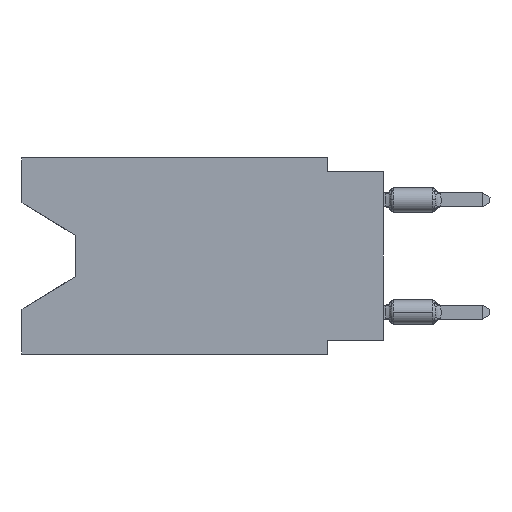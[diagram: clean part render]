
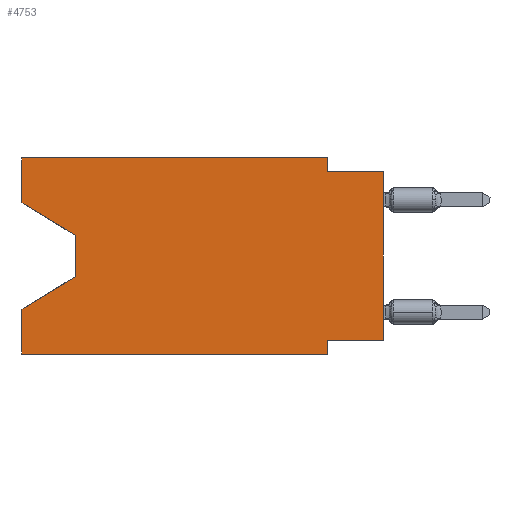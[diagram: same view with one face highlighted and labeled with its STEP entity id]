
A CAD part, left-side view. The second image highlights one B-rep face of the part: STEP entity #4753.
In plain terms, the highlighted planar face has unit normal (-1, 0, 0).
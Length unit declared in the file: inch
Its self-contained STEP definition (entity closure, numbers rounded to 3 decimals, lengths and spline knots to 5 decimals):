
#334 = ORIENTED_EDGE ( 'NONE', *, *, #19707, .F. ) ;
#406 = LINE ( 'NONE', #18886, #5684 ) ;
#440 = ORIENTED_EDGE ( 'NONE', *, *, #2160, .T. ) ;
#480 = VECTOR ( 'NONE', #18942, 39.37008 ) ;
#954 = VERTEX_POINT ( 'NONE', #6726 ) ;
#1253 = ORIENTED_EDGE ( 'NONE', *, *, #10265, .T. ) ;
#1582 = VERTEX_POINT ( 'NONE', #18762 ) ;
#1599 = DIRECTION ( 'NONE',  ( 0., 0., 1. ) ) ;
#1803 = DIRECTION ( 'NONE',  ( 0., -1., 0. ) ) ;
#2113 = DIRECTION ( 'NONE',  ( 0., -0.855, -0.519 ) ) ;
#2151 = VECTOR ( 'NONE', #6159, 39.37008 ) ;
#2160 = EDGE_CURVE ( 'NONE', #17426, #7787, #14604, .T. ) ;
#2364 = ORIENTED_EDGE ( 'NONE', *, *, #13523, .T. ) ;
#2721 = CARTESIAN_POINT ( 'NONE',  ( 0., 0., -0.025 ) ) ;
#3525 = CARTESIAN_POINT ( 'NONE',  ( 0., 0.645, -0.08025 ) ) ;
#3950 = VERTEX_POINT ( 'NONE', #14603 ) ;
#3980 = VERTEX_POINT ( 'NONE', #19431 ) ;
#4102 = VERTEX_POINT ( 'NONE', #10734 ) ;
#4398 = LINE ( 'NONE', #16872, #6889 ) ;
#4489 = DIRECTION ( 'NONE',  ( 1., 0., 0. ) ) ;
#4753 = ADVANCED_FACE ( 'NONE', ( #19963 ), #5931, .F. ) ;
#4955 = VERTEX_POINT ( 'NONE', #7397 ) ;
#5105 = LINE ( 'NONE', #16040, #480 ) ;
#5131 = CARTESIAN_POINT ( 'NONE',  ( 0., 0.645, -0.26975 ) ) ;
#5684 = VECTOR ( 'NONE', #1803, 39.37008 ) ;
#5772 = CARTESIAN_POINT ( 'NONE',  ( 0., 0.55, -0.138 ) ) ;
#5838 = EDGE_CURVE ( 'NONE', #954, #3950, #4398, .T. ) ;
#5931 = PLANE ( 'NONE',  #13612 ) ;
#6133 = CARTESIAN_POINT ( 'NONE',  ( 0., 0., -0.325 ) ) ;
#6159 = DIRECTION ( 'NONE',  ( 0., 0., 1. ) ) ;
#6726 = CARTESIAN_POINT ( 'NONE',  ( 0., 0.645, -0.08025 ) ) ;
#6889 = VECTOR ( 'NONE', #9292, 39.37008 ) ;
#7397 = CARTESIAN_POINT ( 'NONE',  ( 0., 0.1, -0.35 ) ) ;
#7787 = VERTEX_POINT ( 'NONE', #5131 ) ;
#7991 = CARTESIAN_POINT ( 'NONE',  ( 0., 0.55, -0.212 ) ) ;
#8094 = DIRECTION ( 'NONE',  ( 0., 1., 0. ) ) ;
#8268 = VERTEX_POINT ( 'NONE', #15231 ) ;
#8296 = ORIENTED_EDGE ( 'NONE', *, *, #11253, .T. ) ;
#8527 = DIRECTION ( 'NONE',  ( 0., 0., -1. ) ) ;
#8896 = VERTEX_POINT ( 'NONE', #10338 ) ;
#9287 = VERTEX_POINT ( 'NONE', #10129 ) ;
#9292 = DIRECTION ( 'NONE',  ( 0., 0., 1. ) ) ;
#9633 = EDGE_CURVE ( 'NONE', #9796, #8268, #11129, .T. ) ;
#9796 = VERTEX_POINT ( 'NONE', #6133 ) ;
#10129 = CARTESIAN_POINT ( 'NONE',  ( 0., 0.1, -0.025 ) ) ;
#10265 = EDGE_CURVE ( 'NONE', #3980, #4955, #406, .T. ) ;
#10338 = CARTESIAN_POINT ( 'NONE',  ( 0., 0.1, 0. ) ) ;
#10352 = VECTOR ( 'NONE', #19711, 39.37008 ) ;
#10584 = DIRECTION ( 'NONE',  ( 0., 0., -1. ) ) ;
#10616 = CARTESIAN_POINT ( 'NONE',  ( 0., 0.645, 0. ) ) ;
#10715 = LINE ( 'NONE', #15080, #2151 ) ;
#10734 = CARTESIAN_POINT ( 'NONE',  ( 0., 0.55, -0.138 ) ) ;
#11129 = LINE ( 'NONE', #15808, #15724 ) ;
#11253 = EDGE_CURVE ( 'NONE', #9796, #1582, #10715, .T. ) ;
#11554 = LINE ( 'NONE', #16224, #17028 ) ;
#11570 = ORIENTED_EDGE ( 'NONE', *, *, #11752, .F. ) ;
#11752 = EDGE_CURVE ( 'NONE', #8896, #9287, #5105, .T. ) ;
#12025 = ORIENTED_EDGE ( 'NONE', *, *, #14612, .F. ) ;
#12143 = LINE ( 'NONE', #5772, #10352 ) ;
#12288 = CARTESIAN_POINT ( 'NONE',  ( 0., 0.645, 0. ) ) ;
#13153 = VECTOR ( 'NONE', #2113, 39.37008 ) ;
#13290 = CARTESIAN_POINT ( 'NONE',  ( 0., 0.55, -0.212 ) ) ;
#13523 = EDGE_CURVE ( 'NONE', #4102, #17426, #12143, .T. ) ;
#13556 = DIRECTION ( 'NONE',  ( 0., -1., 0. ) ) ;
#13612 = AXIS2_PLACEMENT_3D ( 'NONE', #16570, #4489, #10584 ) ;
#13698 = ORIENTED_EDGE ( 'NONE', *, *, #9633, .F. ) ;
#14603 = CARTESIAN_POINT ( 'NONE',  ( 0., 0.645, 0. ) ) ;
#14604 = LINE ( 'NONE', #13290, #19115 ) ;
#14612 = EDGE_CURVE ( 'NONE', #3980, #7787, #19906, .T. ) ;
#14614 = EDGE_CURVE ( 'NONE', #9287, #1582, #16610, .T. ) ;
#14930 = EDGE_LOOP ( 'NONE', ( #19951, #2364, #440, #12025, #1253, #16631, #13698, #8296, #19456, #11570, #334, #19513 ) ) ;
#15080 = CARTESIAN_POINT ( 'NONE',  ( 0., 0., 0. ) ) ;
#15231 = CARTESIAN_POINT ( 'NONE',  ( 0., 0.1, -0.325 ) ) ;
#15456 = DIRECTION ( 'NONE',  ( 0., -1., 0. ) ) ;
#15724 = VECTOR ( 'NONE', #8094, 39.37008 ) ;
#15808 = CARTESIAN_POINT ( 'NONE',  ( 0., 0., -0.325 ) ) ;
#15907 = VECTOR ( 'NONE', #1599, 39.37008 ) ;
#16040 = CARTESIAN_POINT ( 'NONE',  ( 0., 0.1, 0. ) ) ;
#16224 = CARTESIAN_POINT ( 'NONE',  ( 0., 0.1, -0.35 ) ) ;
#16570 = CARTESIAN_POINT ( 'NONE',  ( 0., 0.645, 0. ) ) ;
#16610 = LINE ( 'NONE', #2721, #17801 ) ;
#16631 = ORIENTED_EDGE ( 'NONE', *, *, #16820, .F. ) ;
#16820 = EDGE_CURVE ( 'NONE', #8268, #4955, #11554, .T. ) ;
#16872 = CARTESIAN_POINT ( 'NONE',  ( 0., 0.645, 0. ) ) ;
#17028 = VECTOR ( 'NONE', #8527, 39.37008 ) ;
#17030 = EDGE_CURVE ( 'NONE', #954, #4102, #19000, .T. ) ;
#17197 = VECTOR ( 'NONE', #15456, 39.37008 ) ;
#17426 = VERTEX_POINT ( 'NONE', #7991 ) ;
#17801 = VECTOR ( 'NONE', #13556, 39.37008 ) ;
#18664 = LINE ( 'NONE', #12288, #17197 ) ;
#18762 = CARTESIAN_POINT ( 'NONE',  ( 0., 0., -0.025 ) ) ;
#18886 = CARTESIAN_POINT ( 'NONE',  ( 0., 0.645, -0.35 ) ) ;
#18942 = DIRECTION ( 'NONE',  ( 0., 0., -1. ) ) ;
#19000 = LINE ( 'NONE', #3525, #13153 ) ;
#19115 = VECTOR ( 'NONE', #19324, 39.37008 ) ;
#19324 = DIRECTION ( 'NONE',  ( 0., 0.855, -0.519 ) ) ;
#19431 = CARTESIAN_POINT ( 'NONE',  ( 0., 0.645, -0.35 ) ) ;
#19456 = ORIENTED_EDGE ( 'NONE', *, *, #14614, .F. ) ;
#19513 = ORIENTED_EDGE ( 'NONE', *, *, #5838, .F. ) ;
#19707 = EDGE_CURVE ( 'NONE', #3950, #8896, #18664, .T. ) ;
#19711 = DIRECTION ( 'NONE',  ( 0., 0., -1. ) ) ;
#19906 = LINE ( 'NONE', #10616, #15907 ) ;
#19951 = ORIENTED_EDGE ( 'NONE', *, *, #17030, .T. ) ;
#19963 = FACE_OUTER_BOUND ( 'NONE', #14930, .T. ) ;
